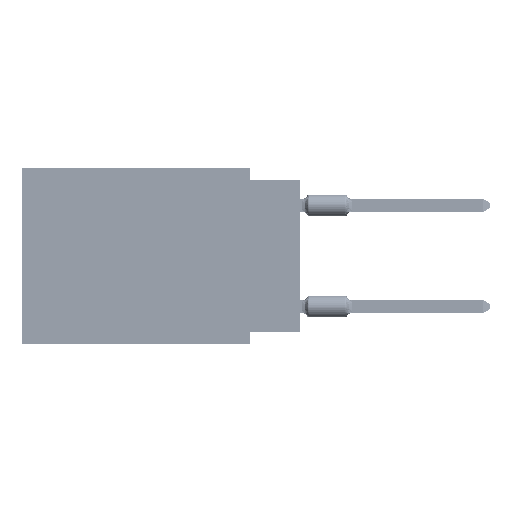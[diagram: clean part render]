
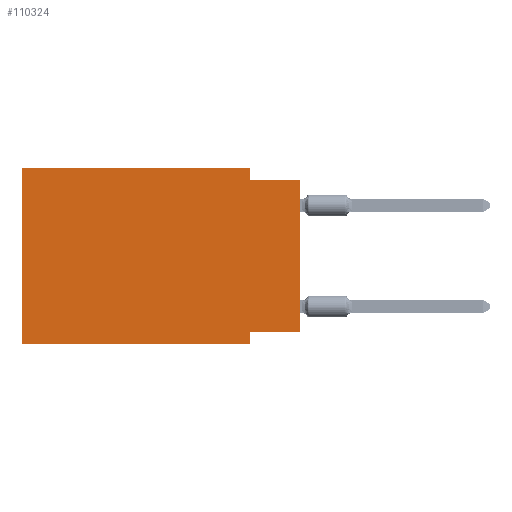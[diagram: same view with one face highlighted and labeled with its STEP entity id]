
A CAD part, left-side view. The second image highlights one B-rep face of the part: STEP entity #110324.
In plain terms, the highlighted planar face has unit normal (-1, 0, 0).
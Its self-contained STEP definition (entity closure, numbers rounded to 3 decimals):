
#289 = VECTOR ( 'NONE', #58479, 1000. ) ;
#1215 = VERTEX_POINT ( 'NONE', #3774 ) ;
#3774 = CARTESIAN_POINT ( 'NONE',  ( 0., 2.54, -0.635 ) ) ;
#9661 = EDGE_CURVE ( 'NONE', #16453, #94426, #24438, .T. ) ;
#12865 = CARTESIAN_POINT ( 'NONE',  ( 0., 0., -8.255 ) ) ;
#13245 = VERTEX_POINT ( 'NONE', #30817 ) ;
#13247 = CARTESIAN_POINT ( 'NONE',  ( 0., 13.97, 0. ) ) ;
#14091 = ORIENTED_EDGE ( 'NONE', *, *, #9661, .F. ) ;
#15782 = EDGE_CURVE ( 'NONE', #102471, #1215, #19505, .T. ) ;
#16453 = VERTEX_POINT ( 'NONE', #82570 ) ;
#19505 = LINE ( 'NONE', #55839, #104390 ) ;
#21097 = EDGE_CURVE ( 'NONE', #83062, #13245, #48990, .T. ) ;
#22307 = LINE ( 'NONE', #40176, #109807 ) ;
#23254 = ORIENTED_EDGE ( 'NONE', *, *, #76318, .T. ) ;
#24438 = LINE ( 'NONE', #95922, #289 ) ;
#29603 = CARTESIAN_POINT ( 'NONE',  ( 0., 0., -0.635 ) ) ;
#30817 = CARTESIAN_POINT ( 'NONE',  ( 0., 13.97, 0. ) ) ;
#31400 = CARTESIAN_POINT ( 'NONE',  ( 0., 13.97, 0. ) ) ;
#31974 = DIRECTION ( 'NONE',  ( 0., -1., 0. ) ) ;
#39467 = DIRECTION ( 'NONE',  ( 1., 0., 0. ) ) ;
#39622 = EDGE_CURVE ( 'NONE', #63641, #16453, #22307, .T. ) ;
#40047 = LINE ( 'NONE', #31400, #43583 ) ;
#40176 = CARTESIAN_POINT ( 'NONE',  ( 0., 0., -8.255 ) ) ;
#43583 = VECTOR ( 'NONE', #31974, 1000. ) ;
#48990 = LINE ( 'NONE', #13247, #68392 ) ;
#50160 = LINE ( 'NONE', #29603, #87113 ) ;
#51137 = ORIENTED_EDGE ( 'NONE', *, *, #21097, .F. ) ;
#52460 = ORIENTED_EDGE ( 'NONE', *, *, #15782, .F. ) ;
#54555 = ORIENTED_EDGE ( 'NONE', *, *, #62302, .F. ) ;
#54688 = DIRECTION ( 'NONE',  ( 0., 0., -1. ) ) ;
#55839 = CARTESIAN_POINT ( 'NONE',  ( 0., 2.54, 0. ) ) ;
#56217 = FACE_OUTER_BOUND ( 'NONE', #65317, .T. ) ;
#57337 = PLANE ( 'NONE',  #73743 ) ;
#58479 = DIRECTION ( 'NONE',  ( 0., 0., -1. ) ) ;
#62302 = EDGE_CURVE ( 'NONE', #1215, #88185, #50160, .T. ) ;
#63641 = VERTEX_POINT ( 'NONE', #12865 ) ;
#65317 = EDGE_LOOP ( 'NONE', ( #23254, #54555, #52460, #84388, #51137, #69714, #14091, #85922 ) ) ;
#65862 = EDGE_CURVE ( 'NONE', #83062, #94426, #98852, .T. ) ;
#68392 = VECTOR ( 'NONE', #80932, 1000. ) ;
#69714 = ORIENTED_EDGE ( 'NONE', *, *, #65862, .T. ) ;
#69989 = CARTESIAN_POINT ( 'NONE',  ( 0., 0., -0.635 ) ) ;
#73486 = DIRECTION ( 'NONE',  ( 0., -1., 0. ) ) ;
#73743 = AXIS2_PLACEMENT_3D ( 'NONE', #91368, #39467, #83288 ) ;
#76100 = DIRECTION ( 'NONE',  ( 0., 0., 1. ) ) ;
#76318 = EDGE_CURVE ( 'NONE', #63641, #88185, #95655, .T. ) ;
#76800 = CARTESIAN_POINT ( 'NONE',  ( 0., 2.54, -8.89 ) ) ;
#80932 = DIRECTION ( 'NONE',  ( 0., 0., 1. ) ) ;
#82570 = CARTESIAN_POINT ( 'NONE',  ( 0., 2.54, -8.255 ) ) ;
#83062 = VERTEX_POINT ( 'NONE', #97430 ) ;
#83288 = DIRECTION ( 'NONE',  ( 0., 0., -1. ) ) ;
#84388 = ORIENTED_EDGE ( 'NONE', *, *, #89259, .F. ) ;
#85335 = DIRECTION ( 'NONE',  ( 0., -1., 0. ) ) ;
#85922 = ORIENTED_EDGE ( 'NONE', *, *, #39622, .F. ) ;
#86451 = CARTESIAN_POINT ( 'NONE',  ( 0., 0., 0. ) ) ;
#87113 = VECTOR ( 'NONE', #85335, 1000. ) ;
#88185 = VERTEX_POINT ( 'NONE', #69989 ) ;
#89259 = EDGE_CURVE ( 'NONE', #13245, #102471, #40047, .T. ) ;
#89637 = CARTESIAN_POINT ( 'NONE',  ( 0., 13.97, -8.89 ) ) ;
#91368 = CARTESIAN_POINT ( 'NONE',  ( 0., 13.97, 0. ) ) ;
#92650 = DIRECTION ( 'NONE',  ( 0., 1., 0. ) ) ;
#94426 = VERTEX_POINT ( 'NONE', #76800 ) ;
#94742 = VECTOR ( 'NONE', #73486, 1000. ) ;
#95655 = LINE ( 'NONE', #86451, #110290 ) ;
#95922 = CARTESIAN_POINT ( 'NONE',  ( 0., 2.54, -8.89 ) ) ;
#97430 = CARTESIAN_POINT ( 'NONE',  ( 0., 13.97, -8.89 ) ) ;
#98852 = LINE ( 'NONE', #89637, #94742 ) ;
#102471 = VERTEX_POINT ( 'NONE', #113073 ) ;
#104390 = VECTOR ( 'NONE', #54688, 1000. ) ;
#109807 = VECTOR ( 'NONE', #92650, 1000. ) ;
#110290 = VECTOR ( 'NONE', #76100, 1000. ) ;
#110324 = ADVANCED_FACE ( 'NONE', ( #56217 ), #57337, .F. ) ;
#113073 = CARTESIAN_POINT ( 'NONE',  ( 0., 2.54, 0. ) ) ;
